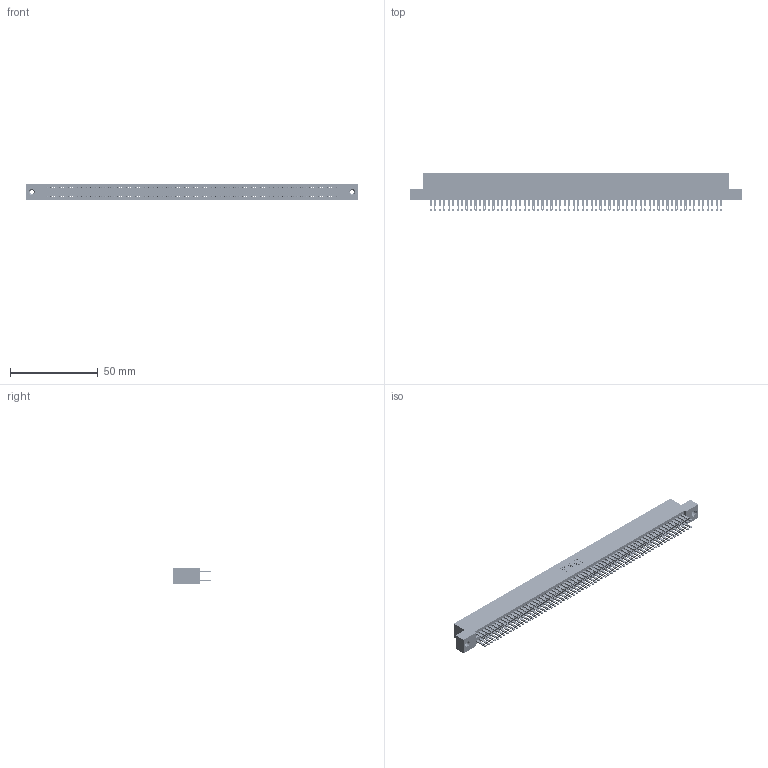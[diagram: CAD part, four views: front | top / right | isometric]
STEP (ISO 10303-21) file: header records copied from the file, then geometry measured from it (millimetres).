
FILE_DESCRIPTION (( 'STEP AP203' ), '1' );
FILE_NAME ('895-132-500-208.STEP', '2020-10-13T17:26:19', ( '' ), ( '' ), 'SwSTEP 2.0', 'SolidWorks 2020', '' );
FILE_SCHEMA (( 'CONFIG_CONTROL_DESIGN' ));
Length unit declared in the file: inch
Products named in the file (4): 845 Part_Flush Mounting Lugs - 0.156 Dia-TI; 345-250-001_345-250-003-102; 895-132-500-208; 345-292-001_345-293-100
Assembly tree (135 placements, depth 2):
  895-132-500-208
    845 Part_Flush Mounting Lugs - 0.156 Dia-TI
    345-292-001_345-293-100  x132
    345-250-001_345-250-003-102  x2
Bounding box: 188.85 x 21.51 x 9.4 mm (x, y, z)
Volume: 18964.6 mm3; surface area: 29857.5 mm2
Topology: 135 solids, 135 shells, 6258 faces, 19089 edges, 12718 vertices
Faces by surface type: plane 3676, cylinder 2566, cone 12, torus 4
Entity records: 49670 total; most frequent: CARTESIAN_POINT 8283, ORIENTED_EDGE 8210, DIRECTION 7303, EDGE_CURVE 4105, VECTOR 3685, LINE 3685, VERTEX_POINT 2732, AXIS2_PLACEMENT_3D 1809
